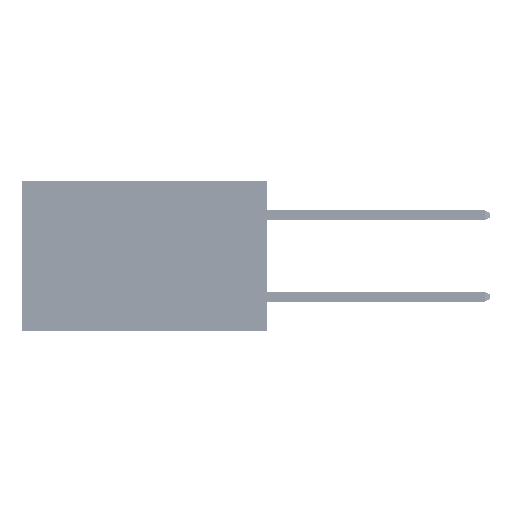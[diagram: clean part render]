
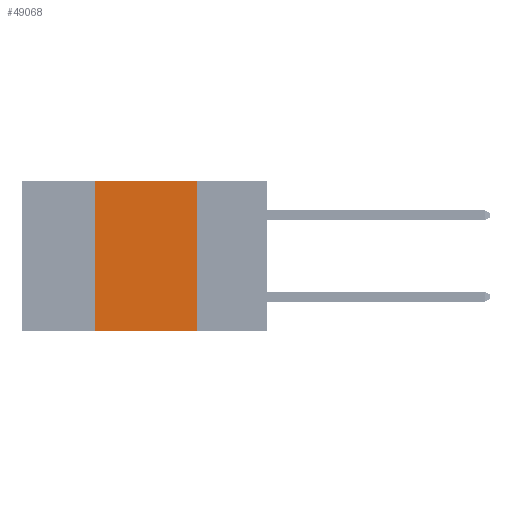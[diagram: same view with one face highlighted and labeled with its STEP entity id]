
A CAD part, left-side view. The second image highlights one B-rep face of the part: STEP entity #49068.
In plain terms, the highlighted planar face has unit normal (-1, 0, 0).
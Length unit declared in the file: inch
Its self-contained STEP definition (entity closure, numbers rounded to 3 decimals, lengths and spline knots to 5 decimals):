
#1842 = VECTOR ( 'NONE', #13341, 39.37008 ) ;
#3164 = FACE_OUTER_BOUND ( 'NONE', #22171, .T. ) ;
#6301 = VECTOR ( 'NONE', #45233, 39.37008 ) ;
#7796 = AXIS2_PLACEMENT_3D ( 'NONE', #11763, #30933, #15375 ) ;
#8133 = VERTEX_POINT ( 'NONE', #19274 ) ;
#8563 = LINE ( 'NONE', #41004, #1842 ) ;
#9319 = EDGE_CURVE ( 'NONE', #25207, #40503, #46712, .T. ) ;
#10551 = LINE ( 'NONE', #33293, #6301 ) ;
#11763 = CARTESIAN_POINT ( 'NONE',  ( 0., 0.6, 0. ) ) ;
#13341 = DIRECTION ( 'NONE',  ( 0., 0., -1. ) ) ;
#14213 = DIRECTION ( 'NONE',  ( 0., -1., 0. ) ) ;
#14917 = VECTOR ( 'NONE', #14213, 39.37008 ) ;
#15235 = CARTESIAN_POINT ( 'NONE',  ( 0., 0.42, -0.37 ) ) ;
#15375 = DIRECTION ( 'NONE',  ( 0., 0., -1. ) ) ;
#19204 = ORIENTED_EDGE ( 'NONE', *, *, #28137, .F. ) ;
#19274 = CARTESIAN_POINT ( 'NONE',  ( 0., 0.42, 0. ) ) ;
#22171 = EDGE_LOOP ( 'NONE', ( #32880, #29997, #19204, #50136 ) ) ;
#22402 = VECTOR ( 'NONE', #48056, 39.37008 ) ;
#25207 = VERTEX_POINT ( 'NONE', #15235 ) ;
#27009 = PLANE ( 'NONE',  #7796 ) ;
#28137 = EDGE_CURVE ( 'NONE', #25207, #8133, #41357, .T. ) ;
#29997 = ORIENTED_EDGE ( 'NONE', *, *, #48073, .F. ) ;
#30933 = DIRECTION ( 'NONE',  ( 1., 0., 0. ) ) ;
#31190 = CARTESIAN_POINT ( 'NONE',  ( 0., 0.17, -0.37 ) ) ;
#32880 = ORIENTED_EDGE ( 'NONE', *, *, #43572, .F. ) ;
#33293 = CARTESIAN_POINT ( 'NONE',  ( 0., 0.6, 0. ) ) ;
#40503 = VERTEX_POINT ( 'NONE', #31190 ) ;
#41004 = CARTESIAN_POINT ( 'NONE',  ( 0., 0.17, 0. ) ) ;
#41079 = VERTEX_POINT ( 'NONE', #49903 ) ;
#41357 = LINE ( 'NONE', #44163, #22402 ) ;
#43572 = EDGE_CURVE ( 'NONE', #41079, #40503, #8563, .T. ) ;
#44163 = CARTESIAN_POINT ( 'NONE',  ( 0., 0.42, 0. ) ) ;
#45233 = DIRECTION ( 'NONE',  ( 0., -1., 0. ) ) ;
#45999 = CARTESIAN_POINT ( 'NONE',  ( 0., 0.6, -0.37 ) ) ;
#46712 = LINE ( 'NONE', #45999, #14917 ) ;
#48056 = DIRECTION ( 'NONE',  ( 0., 0., 1. ) ) ;
#48073 = EDGE_CURVE ( 'NONE', #8133, #41079, #10551, .T. ) ;
#49068 = ADVANCED_FACE ( 'NONE', ( #3164 ), #27009, .F. ) ;
#49903 = CARTESIAN_POINT ( 'NONE',  ( 0., 0.17, 0. ) ) ;
#50136 = ORIENTED_EDGE ( 'NONE', *, *, #9319, .T. ) ;
